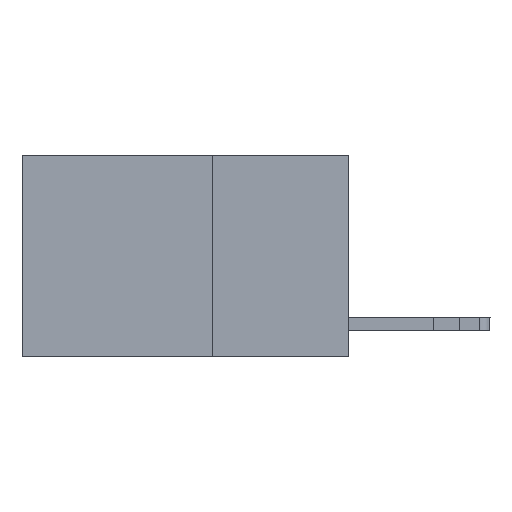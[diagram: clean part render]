
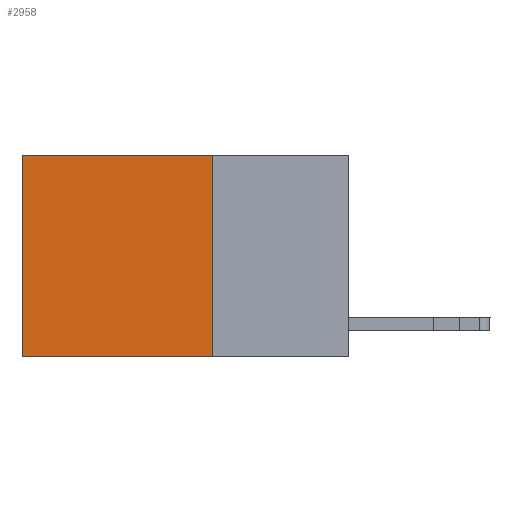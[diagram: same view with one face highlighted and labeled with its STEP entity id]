
A CAD part, left-side view. The second image highlights one B-rep face of the part: STEP entity #2958.
In plain terms, the highlighted planar face has unit normal (-1, 0, 0).
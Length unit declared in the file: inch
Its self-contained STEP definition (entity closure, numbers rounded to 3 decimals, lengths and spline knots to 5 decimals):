
#1075 = VECTOR ( 'NONE', #20339, 39.37008 ) ;
#1119 = EDGE_CURVE ( 'NONE', #9730, #14734, #21228, .T. ) ;
#1297 = AXIS2_PLACEMENT_3D ( 'NONE', #19793, #19581, #19526 ) ;
#1335 = ORIENTED_EDGE ( 'NONE', *, *, #3686, .T. ) ;
#1500 = EDGE_CURVE ( 'NONE', #8837, #10541, #12331, .T. ) ;
#1785 = ORIENTED_EDGE ( 'NONE', *, *, #1119, .T. ) ;
#2248 = VECTOR ( 'NONE', #23045, 39.37008 ) ;
#2614 = DIRECTION ( 'NONE',  ( 0., 1., 0. ) ) ;
#2915 = CARTESIAN_POINT ( 'NONE',  ( 0.2625, 0.6, -0.37 ) ) ;
#2958 = ADVANCED_FACE ( 'NONE', ( #3050 ), #19878, .F. ) ;
#3050 = FACE_OUTER_BOUND ( 'NONE', #20897, .T. ) ;
#3116 = CARTESIAN_POINT ( 'NONE',  ( 0.2625, 0.25, 0. ) ) ;
#3686 = EDGE_CURVE ( 'NONE', #8837, #9730, #7192, .T. ) ;
#3695 = DIRECTION ( 'NONE',  ( 0., 0., -1. ) ) ;
#7192 = LINE ( 'NONE', #3116, #13414 ) ;
#7406 = CARTESIAN_POINT ( 'NONE',  ( 0.2625, 0.6, 0. ) ) ;
#8837 = VERTEX_POINT ( 'NONE', #11746 ) ;
#9730 = VERTEX_POINT ( 'NONE', #24051 ) ;
#10541 = VERTEX_POINT ( 'NONE', #23415 ) ;
#11746 = CARTESIAN_POINT ( 'NONE',  ( 0.2625, 0.25, 0. ) ) ;
#12331 = LINE ( 'NONE', #23993, #16773 ) ;
#12388 = ORIENTED_EDGE ( 'NONE', *, *, #22866, .F. ) ;
#13414 = VECTOR ( 'NONE', #2614, 39.37008 ) ;
#14734 = VERTEX_POINT ( 'NONE', #2915 ) ;
#15515 = CARTESIAN_POINT ( 'NONE',  ( 0.2625, 0.25, -0.37 ) ) ;
#16424 = ORIENTED_EDGE ( 'NONE', *, *, #1500, .F. ) ;
#16773 = VECTOR ( 'NONE', #3695, 39.37008 ) ;
#17385 = LINE ( 'NONE', #15515, #2248 ) ;
#19526 = DIRECTION ( 'NONE',  ( 0., 0., -1. ) ) ;
#19581 = DIRECTION ( 'NONE',  ( 1., 0., 0. ) ) ;
#19793 = CARTESIAN_POINT ( 'NONE',  ( 0.2625, 0.25, 0. ) ) ;
#19878 = PLANE ( 'NONE',  #1297 ) ;
#20339 = DIRECTION ( 'NONE',  ( 0., 0., -1. ) ) ;
#20897 = EDGE_LOOP ( 'NONE', ( #1785, #12388, #16424, #1335 ) ) ;
#21228 = LINE ( 'NONE', #7406, #1075 ) ;
#22866 = EDGE_CURVE ( 'NONE', #10541, #14734, #17385, .T. ) ;
#23045 = DIRECTION ( 'NONE',  ( 0., 1., 0. ) ) ;
#23415 = CARTESIAN_POINT ( 'NONE',  ( 0.2625, 0.25, -0.37 ) ) ;
#23993 = CARTESIAN_POINT ( 'NONE',  ( 0.2625, 0.25, 0. ) ) ;
#24051 = CARTESIAN_POINT ( 'NONE',  ( 0.2625, 0.6, 0. ) ) ;
